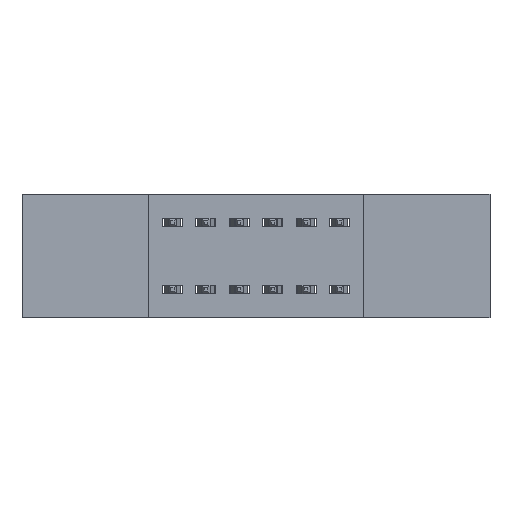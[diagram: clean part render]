
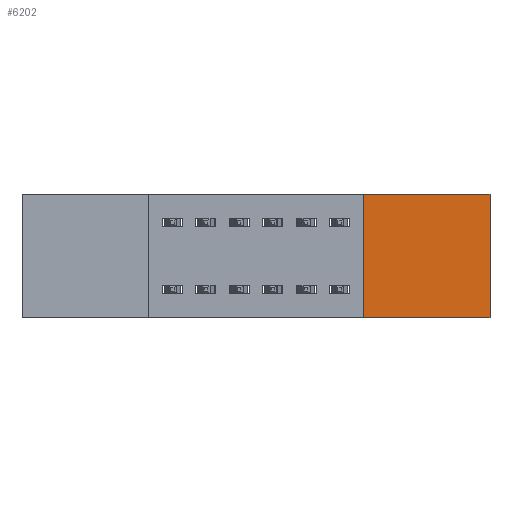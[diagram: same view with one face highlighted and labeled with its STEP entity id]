
A CAD part, front view. The second image highlights one B-rep face of the part: STEP entity #6202.
In plain terms, the highlighted planar face has unit normal (0, -1, 0).
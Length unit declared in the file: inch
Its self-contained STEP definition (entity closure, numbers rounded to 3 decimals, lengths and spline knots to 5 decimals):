
#770 = CARTESIAN_POINT ( 'NONE',  ( 1.023, 0., -0.37 ) ) ;
#1211 = FACE_OUTER_BOUND ( 'NONE', #6806, .T. ) ;
#1229 = EDGE_CURVE ( 'NONE', #3543, #1692, #6936, .T. ) ;
#1436 = CARTESIAN_POINT ( 'NONE',  ( 0., 0., -0.37 ) ) ;
#1459 = DIRECTION ( 'NONE',  ( 0., 0., 1. ) ) ;
#1667 = DIRECTION ( 'NONE',  ( 0., 0., -1. ) ) ;
#1692 = VERTEX_POINT ( 'NONE', #2821 ) ;
#1809 = VECTOR ( 'NONE', #3241, 39.37008 ) ;
#1908 = CARTESIAN_POINT ( 'NONE',  ( 1.4, 0., 0. ) ) ;
#2009 = CARTESIAN_POINT ( 'NONE',  ( 1.023, 0., 0. ) ) ;
#2282 = VERTEX_POINT ( 'NONE', #4478 ) ;
#2476 = VECTOR ( 'NONE', #1459, 39.37008 ) ;
#2643 = CARTESIAN_POINT ( 'NONE',  ( 0., 0., 0. ) ) ;
#2821 = CARTESIAN_POINT ( 'NONE',  ( 1.4, 0., 0. ) ) ;
#3241 = DIRECTION ( 'NONE',  ( 0., 0., -1. ) ) ;
#3278 = VECTOR ( 'NONE', #3308, 39.37008 ) ;
#3308 = DIRECTION ( 'NONE',  ( 1., 0., 0. ) ) ;
#3543 = VERTEX_POINT ( 'NONE', #2009 ) ;
#3616 = AXIS2_PLACEMENT_3D ( 'NONE', #4272, #5587, #1667 ) ;
#3906 = VERTEX_POINT ( 'NONE', #770 ) ;
#3941 = EDGE_CURVE ( 'NONE', #2282, #3906, #4328, .T. ) ;
#4139 = VECTOR ( 'NONE', #6006, 39.37008 ) ;
#4272 = CARTESIAN_POINT ( 'NONE',  ( 0., 0., -0.37 ) ) ;
#4328 = LINE ( 'NONE', #1436, #4139 ) ;
#4478 = CARTESIAN_POINT ( 'NONE',  ( 1.4, 0., -0.37 ) ) ;
#4585 = EDGE_CURVE ( 'NONE', #3906, #3543, #5950, .T. ) ;
#5288 = LINE ( 'NONE', #1908, #1809 ) ;
#5340 = ORIENTED_EDGE ( 'NONE', *, *, #7248, .F. ) ;
#5587 = DIRECTION ( 'NONE',  ( 0., -1., 0. ) ) ;
#5950 = LINE ( 'NONE', #6021, #2476 ) ;
#6006 = DIRECTION ( 'NONE',  ( -1., 0., 0. ) ) ;
#6021 = CARTESIAN_POINT ( 'NONE',  ( 1.023, 0., -0.37 ) ) ;
#6202 = ADVANCED_FACE ( 'NONE', ( #1211 ), #7522, .T. ) ;
#6806 = EDGE_LOOP ( 'NONE', ( #8299, #6903, #5340, #7703 ) ) ;
#6903 = ORIENTED_EDGE ( 'NONE', *, *, #3941, .F. ) ;
#6936 = LINE ( 'NONE', #2643, #3278 ) ;
#7248 = EDGE_CURVE ( 'NONE', #1692, #2282, #5288, .T. ) ;
#7522 = PLANE ( 'NONE',  #3616 ) ;
#7703 = ORIENTED_EDGE ( 'NONE', *, *, #1229, .F. ) ;
#8299 = ORIENTED_EDGE ( 'NONE', *, *, #4585, .F. ) ;
